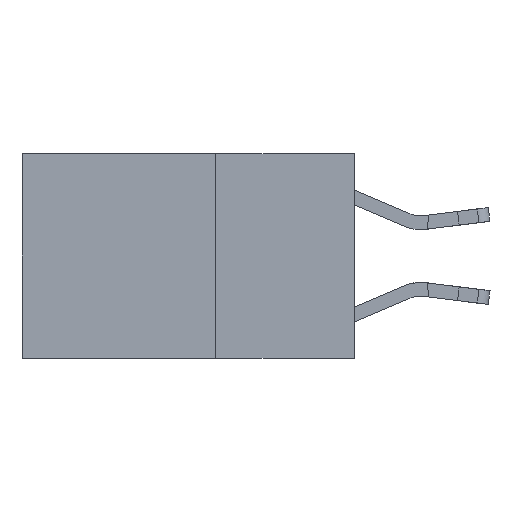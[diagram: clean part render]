
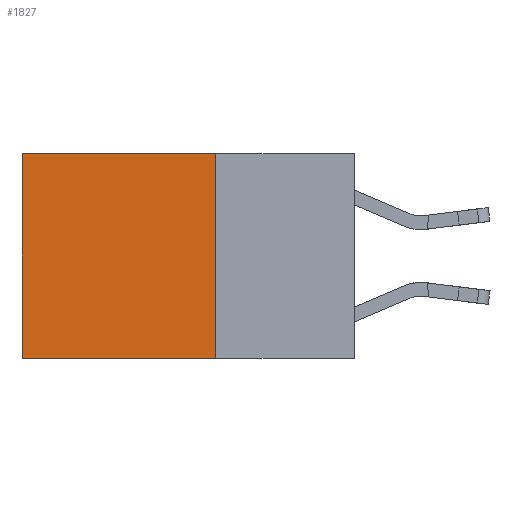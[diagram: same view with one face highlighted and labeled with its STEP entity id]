
A CAD part, left-side view. The second image highlights one B-rep face of the part: STEP entity #1827.
In plain terms, the highlighted planar face has unit normal (-1, 0, 0).
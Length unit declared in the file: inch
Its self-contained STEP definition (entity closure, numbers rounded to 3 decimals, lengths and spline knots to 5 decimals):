
#260 = ORIENTED_EDGE ( 'NONE', *, *, #6762, .T. ) ;
#1319 = DIRECTION ( 'NONE',  ( 0., 0., -1. ) ) ;
#1754 = DIRECTION ( 'NONE',  ( 0., 1., 0. ) ) ;
#1827 = ADVANCED_FACE ( 'NONE', ( #5684 ), #4267, .F. ) ;
#2230 = LINE ( 'NONE', #9106, #13258 ) ;
#2287 = EDGE_CURVE ( 'NONE', #15019, #12533, #2230, .T. ) ;
#2466 = LINE ( 'NONE', #7536, #5488 ) ;
#3021 = CARTESIAN_POINT ( 'NONE',  ( 0.2625, 0.25, 0. ) ) ;
#3545 = EDGE_LOOP ( 'NONE', ( #14007, #12267, #12716, #260 ) ) ;
#4267 = PLANE ( 'NONE',  #9509 ) ;
#4327 = CARTESIAN_POINT ( 'NONE',  ( 0.2625, 0.25, 0. ) ) ;
#4368 = CARTESIAN_POINT ( 'NONE',  ( 0.2625, 0.25, -0.37 ) ) ;
#4970 = VECTOR ( 'NONE', #1754, 39.37008 ) ;
#5488 = VECTOR ( 'NONE', #7364, 39.37008 ) ;
#5684 = FACE_OUTER_BOUND ( 'NONE', #3545, .T. ) ;
#6130 = DIRECTION ( 'NONE',  ( 0., 1., 0. ) ) ;
#6762 = EDGE_CURVE ( 'NONE', #16367, #15019, #9037, .T. ) ;
#7364 = DIRECTION ( 'NONE',  ( 0., 0., -1. ) ) ;
#7536 = CARTESIAN_POINT ( 'NONE',  ( 0.2625, 0.25, 0. ) ) ;
#8601 = VECTOR ( 'NONE', #6130, 39.37008 ) ;
#8774 = CARTESIAN_POINT ( 'NONE',  ( 0.2625, 0.6, -0.37 ) ) ;
#9037 = LINE ( 'NONE', #3021, #4970 ) ;
#9106 = CARTESIAN_POINT ( 'NONE',  ( 0.2625, 0.6, 0. ) ) ;
#9509 = AXIS2_PLACEMENT_3D ( 'NONE', #4327, #14690, #14742 ) ;
#9594 = CARTESIAN_POINT ( 'NONE',  ( 0.2625, 0.6, 0. ) ) ;
#11090 = VERTEX_POINT ( 'NONE', #4368 ) ;
#11311 = EDGE_CURVE ( 'NONE', #11090, #12533, #14126, .T. ) ;
#11511 = CARTESIAN_POINT ( 'NONE',  ( 0.2625, 0.25, -0.37 ) ) ;
#12267 = ORIENTED_EDGE ( 'NONE', *, *, #11311, .F. ) ;
#12533 = VERTEX_POINT ( 'NONE', #8774 ) ;
#12716 = ORIENTED_EDGE ( 'NONE', *, *, #13277, .F. ) ;
#13258 = VECTOR ( 'NONE', #1319, 39.37008 ) ;
#13277 = EDGE_CURVE ( 'NONE', #16367, #11090, #2466, .T. ) ;
#14007 = ORIENTED_EDGE ( 'NONE', *, *, #2287, .T. ) ;
#14126 = LINE ( 'NONE', #11511, #8601 ) ;
#14690 = DIRECTION ( 'NONE',  ( 1., 0., 0. ) ) ;
#14742 = DIRECTION ( 'NONE',  ( 0., 0., -1. ) ) ;
#15019 = VERTEX_POINT ( 'NONE', #9594 ) ;
#15446 = CARTESIAN_POINT ( 'NONE',  ( 0.2625, 0.25, 0. ) ) ;
#16367 = VERTEX_POINT ( 'NONE', #15446 ) ;
